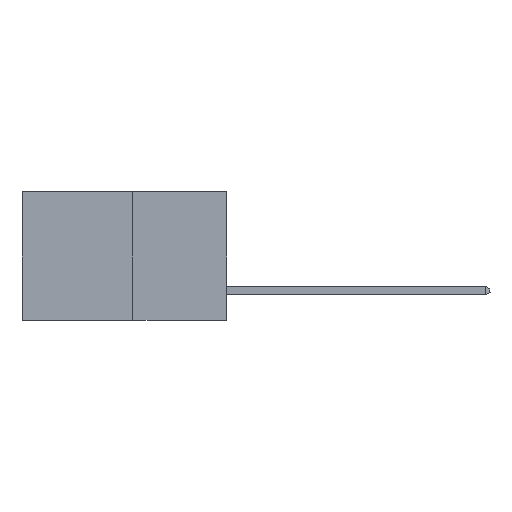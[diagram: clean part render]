
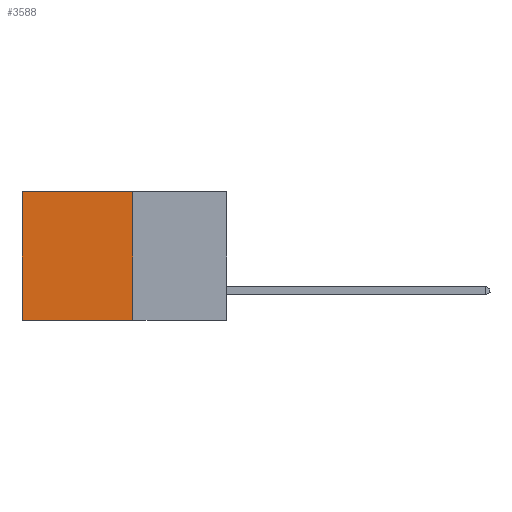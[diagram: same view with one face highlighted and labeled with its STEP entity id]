
A CAD part, left-side view. The second image highlights one B-rep face of the part: STEP entity #3588.
In plain terms, the highlighted planar face has unit normal (-1, 0, 0).
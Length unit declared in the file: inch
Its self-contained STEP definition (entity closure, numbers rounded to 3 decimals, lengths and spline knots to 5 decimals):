
#508 = LINE ( 'NONE', #7926, #4648 ) ;
#1221 = LINE ( 'NONE', #12359, #5961 ) ;
#1304 = AXIS2_PLACEMENT_3D ( 'NONE', #14202, #14124, #14090 ) ;
#1614 = VERTEX_POINT ( 'NONE', #15883 ) ;
#1651 = FACE_OUTER_BOUND ( 'NONE', #11061, .T. ) ;
#3030 = LINE ( 'NONE', #17000, #7199 ) ;
#3588 = ADVANCED_FACE ( 'NONE', ( #1651 ), #14329, .F. ) ;
#3998 = VECTOR ( 'NONE', #14808, 39.37008 ) ;
#4101 = CARTESIAN_POINT ( 'NONE',  ( 0.277, 0.59, -0.37 ) ) ;
#4648 = VECTOR ( 'NONE', #7903, 39.37008 ) ;
#5600 = EDGE_CURVE ( 'NONE', #1614, #11330, #508, .T. ) ;
#5961 = VECTOR ( 'NONE', #20985, 39.37008 ) ;
#7199 = VECTOR ( 'NONE', #16637, 39.37008 ) ;
#7903 = DIRECTION ( 'NONE',  ( 0., 1., 0. ) ) ;
#7926 = CARTESIAN_POINT ( 'NONE',  ( 0.277, 0.27, 0. ) ) ;
#8293 = EDGE_CURVE ( 'NONE', #20563, #13845, #3030, .T. ) ;
#9266 = LINE ( 'NONE', #9629, #3998 ) ;
#9629 = CARTESIAN_POINT ( 'NONE',  ( 0.277, 0.27, -0.37 ) ) ;
#11061 = EDGE_LOOP ( 'NONE', ( #16685, #14344, #11902, #21498 ) ) ;
#11330 = VERTEX_POINT ( 'NONE', #11727 ) ;
#11727 = CARTESIAN_POINT ( 'NONE',  ( 0.277, 0.59, 0. ) ) ;
#11853 = EDGE_CURVE ( 'NONE', #1614, #20563, #9266, .T. ) ;
#11902 = ORIENTED_EDGE ( 'NONE', *, *, #11853, .F. ) ;
#12359 = CARTESIAN_POINT ( 'NONE',  ( 0.277, 0.59, -0.37 ) ) ;
#13845 = VERTEX_POINT ( 'NONE', #4101 ) ;
#13893 = CARTESIAN_POINT ( 'NONE',  ( 0.277, 0.27, -0.37 ) ) ;
#14090 = DIRECTION ( 'NONE',  ( 0., 0., -1. ) ) ;
#14124 = DIRECTION ( 'NONE',  ( 1., 0., 0. ) ) ;
#14202 = CARTESIAN_POINT ( 'NONE',  ( 0.277, 0.27, -0.37 ) ) ;
#14329 = PLANE ( 'NONE',  #1304 ) ;
#14344 = ORIENTED_EDGE ( 'NONE', *, *, #8293, .F. ) ;
#14808 = DIRECTION ( 'NONE',  ( 0., 0., -1. ) ) ;
#15883 = CARTESIAN_POINT ( 'NONE',  ( 0.277, 0.27, 0. ) ) ;
#16637 = DIRECTION ( 'NONE',  ( 0., 1., 0. ) ) ;
#16685 = ORIENTED_EDGE ( 'NONE', *, *, #18757, .T. ) ;
#17000 = CARTESIAN_POINT ( 'NONE',  ( 0.277, 0.27, -0.37 ) ) ;
#18757 = EDGE_CURVE ( 'NONE', #11330, #13845, #1221, .T. ) ;
#20563 = VERTEX_POINT ( 'NONE', #13893 ) ;
#20985 = DIRECTION ( 'NONE',  ( 0., 0., -1. ) ) ;
#21498 = ORIENTED_EDGE ( 'NONE', *, *, #5600, .T. ) ;
